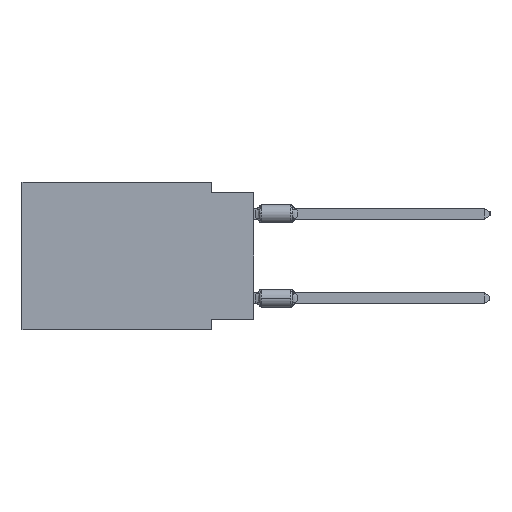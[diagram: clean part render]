
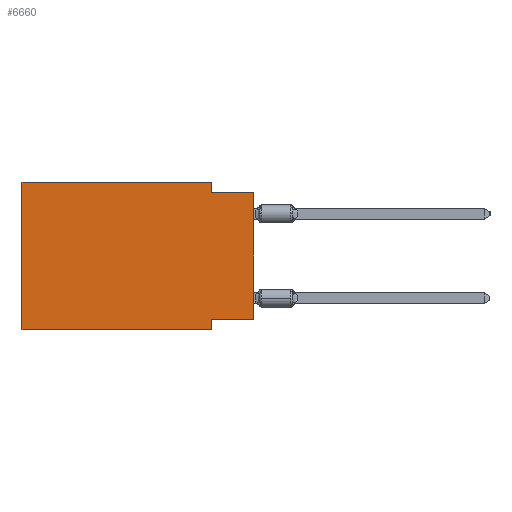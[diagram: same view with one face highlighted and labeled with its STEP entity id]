
A CAD part, left-side view. The second image highlights one B-rep face of the part: STEP entity #6660.
In plain terms, the highlighted planar face has unit normal (-1, 0, 0).
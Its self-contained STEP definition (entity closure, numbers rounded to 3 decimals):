
#463 = DIRECTION ( 'NONE',  ( 0., 0., -1. ) ) ;
#858 = LINE ( 'NONE', #16449, #43677 ) ;
#2137 = LINE ( 'NONE', #44593, #14591 ) ;
#2562 = EDGE_CURVE ( 'NONE', #40311, #19707, #18210, .T. ) ;
#3503 = DIRECTION ( 'NONE',  ( 0., 1., 0. ) ) ;
#4965 = CARTESIAN_POINT ( 'NONE',  ( 0., 2.54, 0. ) ) ;
#5038 = PLANE ( 'NONE',  #37746 ) ;
#6660 = ADVANCED_FACE ( 'NONE', ( #48273 ), #5038, .F. ) ;
#9570 = ORIENTED_EDGE ( 'NONE', *, *, #13528, .F. ) ;
#10435 = VERTEX_POINT ( 'NONE', #29105 ) ;
#11238 = EDGE_CURVE ( 'NONE', #31721, #24423, #858, .T. ) ;
#11268 = LINE ( 'NONE', #49651, #22780 ) ;
#12250 = EDGE_LOOP ( 'NONE', ( #31341, #37004, #25949, #39253, #27096, #14015, #21752, #9570 ) ) ;
#12572 = VECTOR ( 'NONE', #36168, 1000. ) ;
#13528 = EDGE_CURVE ( 'NONE', #37193, #31721, #38045, .T. ) ;
#13665 = LINE ( 'NONE', #29268, #15810 ) ;
#14015 = ORIENTED_EDGE ( 'NONE', *, *, #41325, .T. ) ;
#14081 = VECTOR ( 'NONE', #26674, 1000. ) ;
#14499 = CARTESIAN_POINT ( 'NONE',  ( 0., 0., -8.255 ) ) ;
#14591 = VECTOR ( 'NONE', #29503, 1000. ) ;
#14775 = CARTESIAN_POINT ( 'NONE',  ( 0., 0., -8.255 ) ) ;
#15810 = VECTOR ( 'NONE', #33357, 1000. ) ;
#16449 = CARTESIAN_POINT ( 'NONE',  ( 0., 2.54, -8.89 ) ) ;
#17524 = CARTESIAN_POINT ( 'NONE',  ( 0., 13.97, -8.89 ) ) ;
#17942 = EDGE_CURVE ( 'NONE', #32531, #40311, #2137, .T. ) ;
#18210 = LINE ( 'NONE', #50196, #14081 ) ;
#18289 = EDGE_CURVE ( 'NONE', #10435, #39607, #11268, .T. ) ;
#19268 = CARTESIAN_POINT ( 'NONE',  ( 0., 13.97, 0. ) ) ;
#19707 = VERTEX_POINT ( 'NONE', #24591 ) ;
#21000 = CARTESIAN_POINT ( 'NONE',  ( 0., 2.54, -8.255 ) ) ;
#21752 = ORIENTED_EDGE ( 'NONE', *, *, #11238, .F. ) ;
#22780 = VECTOR ( 'NONE', #33775, 1000. ) ;
#24245 = DIRECTION ( 'NONE',  ( 1., 0., 0. ) ) ;
#24423 = VERTEX_POINT ( 'NONE', #28042 ) ;
#24591 = CARTESIAN_POINT ( 'NONE',  ( 0., 2.54, 0. ) ) ;
#25949 = ORIENTED_EDGE ( 'NONE', *, *, #41363, .F. ) ;
#26674 = DIRECTION ( 'NONE',  ( 0., -1., 0. ) ) ;
#27096 = ORIENTED_EDGE ( 'NONE', *, *, #17942, .F. ) ;
#27304 = CARTESIAN_POINT ( 'NONE',  ( 0., 0., -0.635 ) ) ;
#28042 = CARTESIAN_POINT ( 'NONE',  ( 0., 2.54, -8.89 ) ) ;
#29053 = CARTESIAN_POINT ( 'NONE',  ( 0., 0., 0. ) ) ;
#29105 = CARTESIAN_POINT ( 'NONE',  ( 0., 2.54, -0.635 ) ) ;
#29268 = CARTESIAN_POINT ( 'NONE',  ( 0., 13.97, -8.89 ) ) ;
#29503 = DIRECTION ( 'NONE',  ( 0., 0., 1. ) ) ;
#30710 = VECTOR ( 'NONE', #37469, 1000. ) ;
#31341 = ORIENTED_EDGE ( 'NONE', *, *, #45215, .T. ) ;
#31721 = VERTEX_POINT ( 'NONE', #21000 ) ;
#32531 = VERTEX_POINT ( 'NONE', #17524 ) ;
#33357 = DIRECTION ( 'NONE',  ( 0., -1., 0. ) ) ;
#33387 = LINE ( 'NONE', #29053, #30710 ) ;
#33775 = DIRECTION ( 'NONE',  ( 0., -1., 0. ) ) ;
#36168 = DIRECTION ( 'NONE',  ( 0., 0., -1. ) ) ;
#36389 = DIRECTION ( 'NONE',  ( 0., 0., -1. ) ) ;
#37004 = ORIENTED_EDGE ( 'NONE', *, *, #18289, .F. ) ;
#37184 = LINE ( 'NONE', #4965, #12572 ) ;
#37193 = VERTEX_POINT ( 'NONE', #14499 ) ;
#37469 = DIRECTION ( 'NONE',  ( 0., 0., 1. ) ) ;
#37746 = AXIS2_PLACEMENT_3D ( 'NONE', #43193, #24245, #463 ) ;
#38045 = LINE ( 'NONE', #14775, #41398 ) ;
#39253 = ORIENTED_EDGE ( 'NONE', *, *, #2562, .F. ) ;
#39607 = VERTEX_POINT ( 'NONE', #27304 ) ;
#40311 = VERTEX_POINT ( 'NONE', #19268 ) ;
#41325 = EDGE_CURVE ( 'NONE', #32531, #24423, #13665, .T. ) ;
#41363 = EDGE_CURVE ( 'NONE', #19707, #10435, #37184, .T. ) ;
#41398 = VECTOR ( 'NONE', #3503, 1000. ) ;
#43193 = CARTESIAN_POINT ( 'NONE',  ( 0., 13.97, 0. ) ) ;
#43677 = VECTOR ( 'NONE', #36389, 1000. ) ;
#44593 = CARTESIAN_POINT ( 'NONE',  ( 0., 13.97, 0. ) ) ;
#45215 = EDGE_CURVE ( 'NONE', #37193, #39607, #33387, .T. ) ;
#48273 = FACE_OUTER_BOUND ( 'NONE', #12250, .T. ) ;
#49651 = CARTESIAN_POINT ( 'NONE',  ( 0., 0., -0.635 ) ) ;
#50196 = CARTESIAN_POINT ( 'NONE',  ( 0., 13.97, 0. ) ) ;
